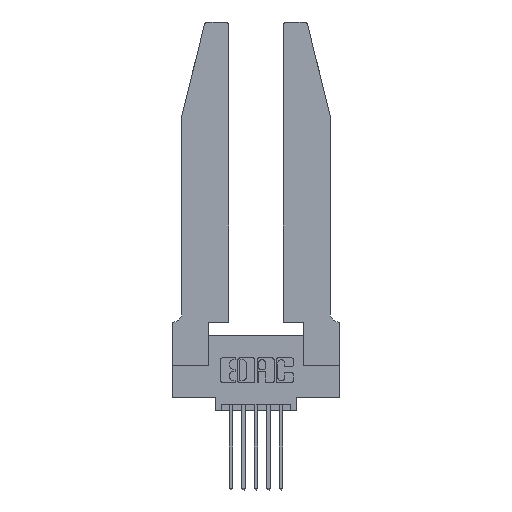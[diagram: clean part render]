
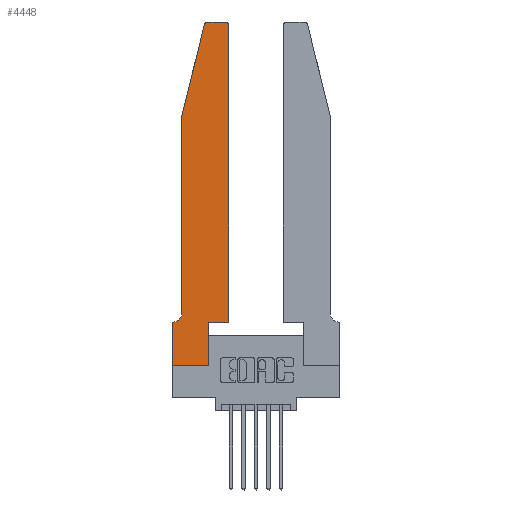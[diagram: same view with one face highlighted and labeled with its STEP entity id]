
A CAD part, top view. The second image highlights one B-rep face of the part: STEP entity #4448.
In plain terms, the highlighted planar face has unit normal (0, 0, 1).
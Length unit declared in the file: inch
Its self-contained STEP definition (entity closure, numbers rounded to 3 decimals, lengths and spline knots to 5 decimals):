
#14 = LINE ( 'NONE', #8461, #10594 ) ;
#43 = CARTESIAN_POINT ( 'NONE',  ( 0.4505, 2.72, 0.37 ) ) ;
#91 = VERTEX_POINT ( 'NONE', #10378 ) ;
#103 = CARTESIAN_POINT ( 'NONE',  ( 0.4505, 0.35, 0.37 ) ) ;
#302 = VERTEX_POINT ( 'NONE', #4199 ) ;
#571 = CARTESIAN_POINT ( 'NONE',  ( 0.0755, 2., 0.37 ) ) ;
#706 = EDGE_CURVE ( 'NONE', #7163, #8276, #4564, .T. ) ;
#1329 = VERTEX_POINT ( 'NONE', #3660 ) ;
#1782 = ORIENTED_EDGE ( 'NONE', *, *, #12607, .T. ) ;
#1801 = EDGE_CURVE ( 'NONE', #4443, #302, #6313, .T. ) ;
#1902 = VECTOR ( 'NONE', #3594, 39.37008 ) ;
#1949 = VECTOR ( 'NONE', #3443, 39.37008 ) ;
#2066 = LINE ( 'NONE', #3353, #12890 ) ;
#2305 = VERTEX_POINT ( 'NONE', #103 ) ;
#2672 = EDGE_CURVE ( 'NONE', #6696, #3131, #8825, .T. ) ;
#2730 = ORIENTED_EDGE ( 'NONE', *, *, #8281, .T. ) ;
#2819 = AXIS2_PLACEMENT_3D ( 'NONE', #5619, #5603, #5601 ) ;
#2894 = ORIENTED_EDGE ( 'NONE', *, *, #10813, .T. ) ;
#3124 = DIRECTION ( 'NONE',  ( -0.239, -0.971, 0. ) ) ;
#3131 = VERTEX_POINT ( 'NONE', #5293 ) ;
#3324 = VECTOR ( 'NONE', #4961, 39.37008 ) ;
#3353 = CARTESIAN_POINT ( 'NONE',  ( 0., 0., 0.37 ) ) ;
#3443 = DIRECTION ( 'NONE',  ( 1., 0., 0. ) ) ;
#3530 = VECTOR ( 'NONE', #11721, 39.37008 ) ;
#3594 = DIRECTION ( 'NONE',  ( 0., 1., 0. ) ) ;
#3660 = CARTESIAN_POINT ( 'NONE',  ( 0.2865, 0., 0.37 ) ) ;
#4195 = ORIENTED_EDGE ( 'NONE', *, *, #1801, .T. ) ;
#4199 = CARTESIAN_POINT ( 'NONE',  ( 0., 0.35, 0.37 ) ) ;
#4260 = LINE ( 'NONE', #5688, #3530 ) ;
#4373 = ORIENTED_EDGE ( 'NONE', *, *, #706, .T. ) ;
#4443 = VERTEX_POINT ( 'NONE', #9811 ) ;
#4448 = ADVANCED_FACE ( 'NONE', ( #12483 ), #10301, .T. ) ;
#4564 = LINE ( 'NONE', #571, #9746 ) ;
#4678 = LINE ( 'NONE', #9743, #1949 ) ;
#4777 = DIRECTION ( 'NONE',  ( 0., 0., 1. ) ) ;
#4814 = CARTESIAN_POINT ( 'NONE',  ( 0., 0., 0.37 ) ) ;
#4868 = VERTEX_POINT ( 'NONE', #13453 ) ;
#4961 = DIRECTION ( 'NONE',  ( -1., 0., 0. ) ) ;
#5293 = CARTESIAN_POINT ( 'NONE',  ( 0.4205, 2.75, 0.37 ) ) ;
#5601 = DIRECTION ( 'NONE',  ( -1., 0., 0. ) ) ;
#5603 = DIRECTION ( 'NONE',  ( 0., 0., -1. ) ) ;
#5619 = CARTESIAN_POINT ( 'NONE',  ( 0.0055, 0.42, 0.37 ) ) ;
#5651 = VERTEX_POINT ( 'NONE', #6888 ) ;
#5688 = CARTESIAN_POINT ( 'NONE',  ( 0.2605, 2.75, 0.37 ) ) ;
#5759 = CARTESIAN_POINT ( 'NONE',  ( 0.284, 2.75, 0.37 ) ) ;
#5835 = EDGE_CURVE ( 'NONE', #8276, #4443, #8622, .T. ) ;
#6148 = ORIENTED_EDGE ( 'NONE', *, *, #8897, .T. ) ;
#6313 = LINE ( 'NONE', #13043, #3324 ) ;
#6322 = EDGE_LOOP ( 'NONE', ( #9099, #1782, #2894, #4373, #13436, #4195, #2730, #8993, #7586, #6148, #6986, #12875 ) ) ;
#6497 = CIRCLE ( 'NONE', #7290, 0.03 ) ;
#6696 = VERTEX_POINT ( 'NONE', #43 ) ;
#6852 = AXIS2_PLACEMENT_3D ( 'NONE', #11266, #13306, #11121 ) ;
#6888 = CARTESIAN_POINT ( 'NONE',  ( 0.2865, 0.35, 0.37 ) ) ;
#6960 = AXIS2_PLACEMENT_3D ( 'NONE', #10345, #7391, #9615 ) ;
#6986 = ORIENTED_EDGE ( 'NONE', *, *, #10149, .T. ) ;
#7163 = VERTEX_POINT ( 'NONE', #11714 ) ;
#7290 = AXIS2_PLACEMENT_3D ( 'NONE', #10928, #4777, #11910 ) ;
#7391 = DIRECTION ( 'NONE',  ( 0., 0., 1. ) ) ;
#7586 = ORIENTED_EDGE ( 'NONE', *, *, #11050, .T. ) ;
#7636 = LINE ( 'NONE', #9455, #12275 ) ;
#7856 = VERTEX_POINT ( 'NONE', #5759 ) ;
#7906 = EDGE_CURVE ( 'NONE', #91, #1329, #9638, .T. ) ;
#8276 = VERTEX_POINT ( 'NONE', #11670 ) ;
#8281 = EDGE_CURVE ( 'NONE', #302, #91, #2066, .T. ) ;
#8461 = CARTESIAN_POINT ( 'NONE',  ( 0.0755, 2., 0.37 ) ) ;
#8622 = CIRCLE ( 'NONE', #2819, 0.07 ) ;
#8825 = CIRCLE ( 'NONE', #6852, 0.03 ) ;
#8897 = EDGE_CURVE ( 'NONE', #5651, #2305, #4678, .T. ) ;
#8993 = ORIENTED_EDGE ( 'NONE', *, *, #7906, .T. ) ;
#9099 = ORIENTED_EDGE ( 'NONE', *, *, #12070, .T. ) ;
#9326 = VECTOR ( 'NONE', #10960, 39.37008 ) ;
#9455 = CARTESIAN_POINT ( 'NONE',  ( 0.4505, 0.35, 0.37 ) ) ;
#9615 = DIRECTION ( 'NONE',  ( 1., 0., 0. ) ) ;
#9638 = LINE ( 'NONE', #4814, #9326 ) ;
#9743 = CARTESIAN_POINT ( 'NONE',  ( 0.4505, 0.35, 0.37 ) ) ;
#9746 = VECTOR ( 'NONE', #11491, 39.37008 ) ;
#9811 = CARTESIAN_POINT ( 'NONE',  ( 0.0055, 0.35, 0.37 ) ) ;
#10149 = EDGE_CURVE ( 'NONE', #2305, #6696, #7636, .T. ) ;
#10301 = PLANE ( 'NONE',  #6960 ) ;
#10345 = CARTESIAN_POINT ( 'NONE',  ( 0., 0.35, 0.37 ) ) ;
#10378 = CARTESIAN_POINT ( 'NONE',  ( 0., 0., 0.37 ) ) ;
#10449 = DIRECTION ( 'NONE',  ( 0., 1., 0. ) ) ;
#10594 = VECTOR ( 'NONE', #3124, 39.37008 ) ;
#10813 = EDGE_CURVE ( 'NONE', #4868, #7163, #14, .T. ) ;
#10928 = CARTESIAN_POINT ( 'NONE',  ( 0.284, 2.72, 0.37 ) ) ;
#10960 = DIRECTION ( 'NONE',  ( 1., 0., 0. ) ) ;
#11050 = EDGE_CURVE ( 'NONE', #1329, #5651, #13055, .T. ) ;
#11121 = DIRECTION ( 'NONE',  ( 1., 0., 0. ) ) ;
#11266 = CARTESIAN_POINT ( 'NONE',  ( 0.4205, 2.72, 0.37 ) ) ;
#11491 = DIRECTION ( 'NONE',  ( 0., -1., 0. ) ) ;
#11670 = CARTESIAN_POINT ( 'NONE',  ( 0.0755, 0.42, 0.37 ) ) ;
#11714 = CARTESIAN_POINT ( 'NONE',  ( 0.0755, 2., 0.37 ) ) ;
#11721 = DIRECTION ( 'NONE',  ( -1., 0., 0. ) ) ;
#11907 = CARTESIAN_POINT ( 'NONE',  ( 0.2865, 0.35, 0.37 ) ) ;
#11910 = DIRECTION ( 'NONE',  ( 1., 0., 0. ) ) ;
#12070 = EDGE_CURVE ( 'NONE', #3131, #7856, #4260, .T. ) ;
#12275 = VECTOR ( 'NONE', #10449, 39.37008 ) ;
#12483 = FACE_OUTER_BOUND ( 'NONE', #6322, .T. ) ;
#12607 = EDGE_CURVE ( 'NONE', #7856, #4868, #6497, .T. ) ;
#12875 = ORIENTED_EDGE ( 'NONE', *, *, #2672, .T. ) ;
#12890 = VECTOR ( 'NONE', #13663, 39.37008 ) ;
#13043 = CARTESIAN_POINT ( 'NONE',  ( 0.0755, 0.35, 0.37 ) ) ;
#13055 = LINE ( 'NONE', #11907, #1902 ) ;
#13306 = DIRECTION ( 'NONE',  ( 0., 0., 1. ) ) ;
#13436 = ORIENTED_EDGE ( 'NONE', *, *, #5835, .T. ) ;
#13453 = CARTESIAN_POINT ( 'NONE',  ( 0.25487, 2.72718, 0.37 ) ) ;
#13663 = DIRECTION ( 'NONE',  ( 0., -1., 0. ) ) ;
